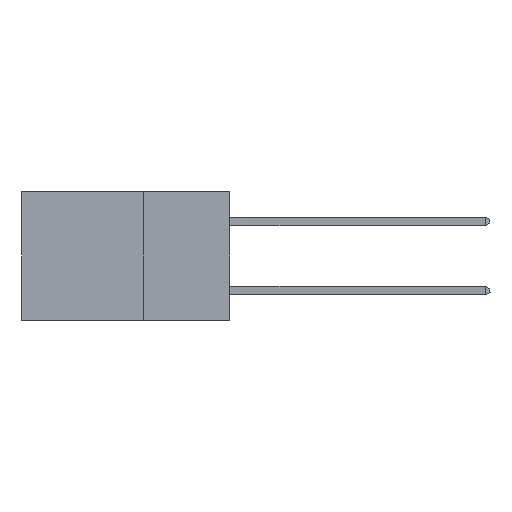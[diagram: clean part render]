
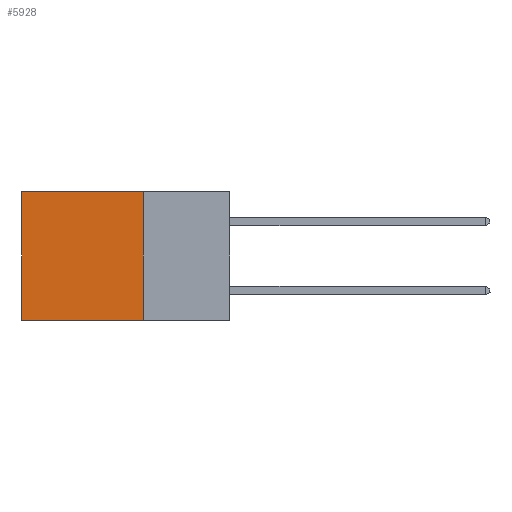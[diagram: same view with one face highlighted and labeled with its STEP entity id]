
A CAD part, left-side view. The second image highlights one B-rep face of the part: STEP entity #5928.
In plain terms, the highlighted planar face has unit normal (-1, 0, 0).
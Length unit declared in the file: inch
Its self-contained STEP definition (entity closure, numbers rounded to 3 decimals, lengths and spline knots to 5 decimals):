
#1333 = LINE ( 'NONE', #2601, #11602 ) ;
#2601 = CARTESIAN_POINT ( 'NONE',  ( 0.298, 0.25, 0. ) ) ;
#3982 = DIRECTION ( 'NONE',  ( 0., 0., -1. ) ) ;
#4231 = ORIENTED_EDGE ( 'NONE', *, *, #12178, .F. ) ;
#4292 = EDGE_CURVE ( 'NONE', #5920, #9266, #11721, .T. ) ;
#5008 = FACE_OUTER_BOUND ( 'NONE', #18680, .T. ) ;
#5222 = LINE ( 'NONE', #9643, #17923 ) ;
#5297 = CARTESIAN_POINT ( 'NONE',  ( 0.298, 0.25, 0. ) ) ;
#5920 = VERTEX_POINT ( 'NONE', #8742 ) ;
#5928 = ADVANCED_FACE ( 'NONE', ( #5008 ), #7395, .F. ) ;
#6929 = AXIS2_PLACEMENT_3D ( 'NONE', #17553, #8868, #7460 ) ;
#7190 = ORIENTED_EDGE ( 'NONE', *, *, #10643, .F. ) ;
#7395 = PLANE ( 'NONE',  #6929 ) ;
#7460 = DIRECTION ( 'NONE',  ( 0., 0., -1. ) ) ;
#7849 = VERTEX_POINT ( 'NONE', #14183 ) ;
#8642 = CARTESIAN_POINT ( 'NONE',  ( 0.298, 0.25, -0.37 ) ) ;
#8679 = VECTOR ( 'NONE', #15758, 39.37008 ) ;
#8742 = CARTESIAN_POINT ( 'NONE',  ( 0.298, 0.25, 0. ) ) ;
#8868 = DIRECTION ( 'NONE',  ( 1., 0., 0. ) ) ;
#9266 = VERTEX_POINT ( 'NONE', #11191 ) ;
#9522 = DIRECTION ( 'NONE',  ( 0., 0., -1. ) ) ;
#9643 = CARTESIAN_POINT ( 'NONE',  ( 0.298, 0.6, 0. ) ) ;
#9836 = LINE ( 'NONE', #8642, #8679 ) ;
#10638 = VERTEX_POINT ( 'NONE', #12799 ) ;
#10643 = EDGE_CURVE ( 'NONE', #10638, #7849, #9836, .T. ) ;
#11191 = CARTESIAN_POINT ( 'NONE',  ( 0.298, 0.6, 0. ) ) ;
#11303 = ORIENTED_EDGE ( 'NONE', *, *, #4292, .T. ) ;
#11602 = VECTOR ( 'NONE', #3982, 39.37008 ) ;
#11628 = EDGE_CURVE ( 'NONE', #9266, #7849, #5222, .T. ) ;
#11721 = LINE ( 'NONE', #5297, #12403 ) ;
#11882 = ORIENTED_EDGE ( 'NONE', *, *, #11628, .T. ) ;
#12178 = EDGE_CURVE ( 'NONE', #5920, #10638, #1333, .T. ) ;
#12403 = VECTOR ( 'NONE', #17122, 39.37008 ) ;
#12799 = CARTESIAN_POINT ( 'NONE',  ( 0.298, 0.25, -0.37 ) ) ;
#14183 = CARTESIAN_POINT ( 'NONE',  ( 0.298, 0.6, -0.37 ) ) ;
#15758 = DIRECTION ( 'NONE',  ( 0., 1., 0. ) ) ;
#17122 = DIRECTION ( 'NONE',  ( 0., 1., 0. ) ) ;
#17553 = CARTESIAN_POINT ( 'NONE',  ( 0.298, 0.25, 0. ) ) ;
#17923 = VECTOR ( 'NONE', #9522, 39.37008 ) ;
#18680 = EDGE_LOOP ( 'NONE', ( #11882, #7190, #4231, #11303 ) ) ;
